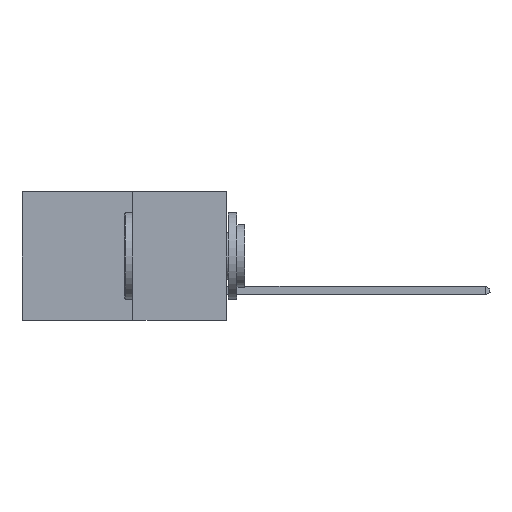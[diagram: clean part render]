
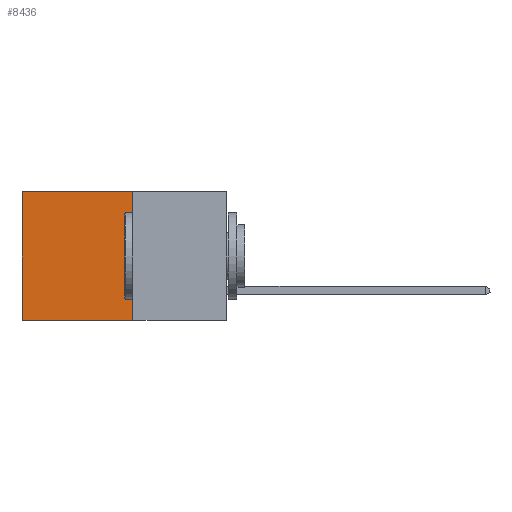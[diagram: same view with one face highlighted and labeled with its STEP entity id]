
A CAD part, left-side view. The second image highlights one B-rep face of the part: STEP entity #8436.
In plain terms, the highlighted planar face has unit normal (-1, 0, 0).
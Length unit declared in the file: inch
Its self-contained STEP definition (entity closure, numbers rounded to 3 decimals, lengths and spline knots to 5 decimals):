
#188 = ORIENTED_EDGE ( 'NONE', *, *, #4479, .F. ) ;
#1044 = LINE ( 'NONE', #17124, #16951 ) ;
#1980 = VECTOR ( 'NONE', #5290, 39.37008 ) ;
#3289 = DIRECTION ( 'NONE',  ( 0., 0., -1. ) ) ;
#4145 = ORIENTED_EDGE ( 'NONE', *, *, #6512, .F. ) ;
#4479 = EDGE_CURVE ( 'NONE', #9475, #15671, #9903, .T. ) ;
#4783 = AXIS2_PLACEMENT_3D ( 'NONE', #5183, #4924, #4899 ) ;
#4899 = DIRECTION ( 'NONE',  ( 0., 0., -1. ) ) ;
#4924 = DIRECTION ( 'NONE',  ( 1., 0., 0. ) ) ;
#5007 = PLANE ( 'NONE',  #4783 ) ;
#5183 = CARTESIAN_POINT ( 'NONE',  ( 0.277, 0.27, -0.37 ) ) ;
#5290 = DIRECTION ( 'NONE',  ( 0., 0., -1. ) ) ;
#5496 = CARTESIAN_POINT ( 'NONE',  ( 0.277, 0.27, -0.37 ) ) ;
#5976 = FACE_OUTER_BOUND ( 'NONE', #18383, .T. ) ;
#6512 = EDGE_CURVE ( 'NONE', #9682, #9475, #9573, .T. ) ;
#6771 = CARTESIAN_POINT ( 'NONE',  ( 0.277, 0.27, -0.37 ) ) ;
#6798 = DIRECTION ( 'NONE',  ( 0., 1., 0. ) ) ;
#7017 = EDGE_CURVE ( 'NONE', #9682, #15347, #1044, .T. ) ;
#7827 = CARTESIAN_POINT ( 'NONE',  ( 0.277, 0.59, -0.37 ) ) ;
#8436 = ADVANCED_FACE ( 'NONE', ( #5976 ), #5007, .F. ) ;
#8682 = ORIENTED_EDGE ( 'NONE', *, *, #7017, .T. ) ;
#9475 = VERTEX_POINT ( 'NONE', #15202 ) ;
#9484 = VECTOR ( 'NONE', #3289, 39.37008 ) ;
#9573 = LINE ( 'NONE', #5496, #1980 ) ;
#9682 = VERTEX_POINT ( 'NONE', #11197 ) ;
#9903 = LINE ( 'NONE', #6771, #17717 ) ;
#10937 = EDGE_CURVE ( 'NONE', #15347, #15671, #13456, .T. ) ;
#11197 = CARTESIAN_POINT ( 'NONE',  ( 0.277, 0.27, 0. ) ) ;
#13456 = LINE ( 'NONE', #7827, #9484 ) ;
#15202 = CARTESIAN_POINT ( 'NONE',  ( 0.277, 0.27, -0.37 ) ) ;
#15347 = VERTEX_POINT ( 'NONE', #16241 ) ;
#15671 = VERTEX_POINT ( 'NONE', #18416 ) ;
#16241 = CARTESIAN_POINT ( 'NONE',  ( 0.277, 0.59, 0. ) ) ;
#16951 = VECTOR ( 'NONE', #17148, 39.37008 ) ;
#17124 = CARTESIAN_POINT ( 'NONE',  ( 0.277, 0.27, 0. ) ) ;
#17148 = DIRECTION ( 'NONE',  ( 0., 1., 0. ) ) ;
#17717 = VECTOR ( 'NONE', #6798, 39.37008 ) ;
#18383 = EDGE_LOOP ( 'NONE', ( #18588, #188, #4145, #8682 ) ) ;
#18416 = CARTESIAN_POINT ( 'NONE',  ( 0.277, 0.59, -0.37 ) ) ;
#18588 = ORIENTED_EDGE ( 'NONE', *, *, #10937, .T. ) ;
